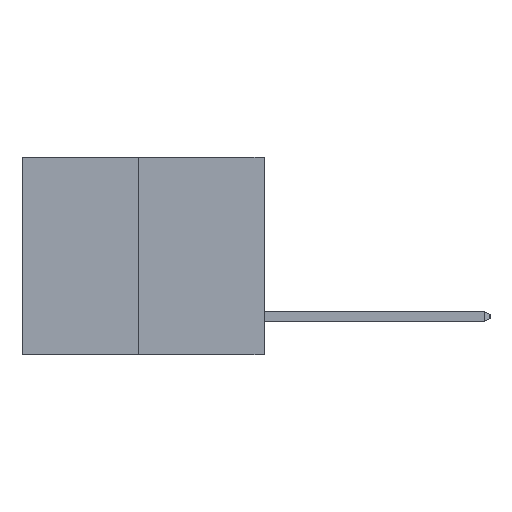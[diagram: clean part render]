
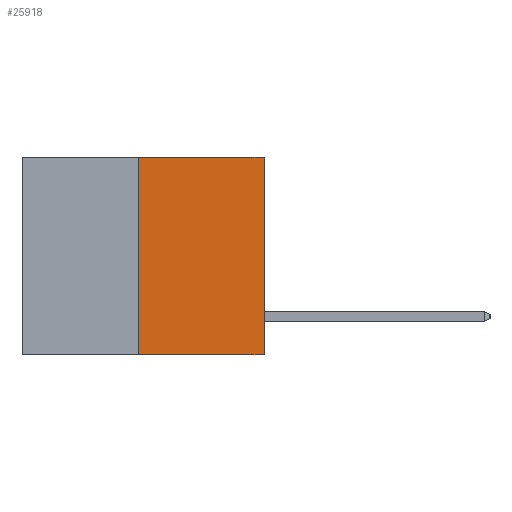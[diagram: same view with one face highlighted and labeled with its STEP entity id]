
A CAD part, left-side view. The second image highlights one B-rep face of the part: STEP entity #25918.
In plain terms, the highlighted planar face has unit normal (-1, 0, 0).
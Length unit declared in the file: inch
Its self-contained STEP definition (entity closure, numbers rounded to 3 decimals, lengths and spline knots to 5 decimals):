
#347 = EDGE_CURVE ( 'NONE', #13254, #6863, #13673, .T. ) ;
#602 = EDGE_CURVE ( 'NONE', #24014, #6863, #19933, .T. ) ;
#3630 = FACE_OUTER_BOUND ( 'NONE', #6779, .T. ) ;
#3712 = CARTESIAN_POINT ( 'NONE',  ( 0., 0.6, -0.49 ) ) ;
#3800 = VECTOR ( 'NONE', #10921, 39.37008 ) ;
#4757 = CARTESIAN_POINT ( 'NONE',  ( 0., 0., 0. ) ) ;
#5006 = CARTESIAN_POINT ( 'NONE',  ( 0., 0.312, 0. ) ) ;
#5652 = PLANE ( 'NONE',  #18351 ) ;
#6779 = EDGE_LOOP ( 'NONE', ( #8605, #16521, #17600, #12822 ) ) ;
#6863 = VERTEX_POINT ( 'NONE', #4757 ) ;
#7067 = CARTESIAN_POINT ( 'NONE',  ( 0., 0.312, -0.49 ) ) ;
#7430 = VECTOR ( 'NONE', #17820, 39.37008 ) ;
#7860 = DIRECTION ( 'NONE',  ( 0., -1., 0. ) ) ;
#8605 = ORIENTED_EDGE ( 'NONE', *, *, #10778, .F. ) ;
#9129 = DIRECTION ( 'NONE',  ( 0., -1., 0. ) ) ;
#10778 = EDGE_CURVE ( 'NONE', #15456, #24014, #16385, .T. ) ;
#10921 = DIRECTION ( 'NONE',  ( 0., 0., 1. ) ) ;
#11393 = CARTESIAN_POINT ( 'NONE',  ( 0., 0.6, 0. ) ) ;
#11877 = CARTESIAN_POINT ( 'NONE',  ( 0., 0., -0.49 ) ) ;
#11909 = DIRECTION ( 'NONE',  ( 0., 0., -1. ) ) ;
#12227 = EDGE_CURVE ( 'NONE', #15456, #13254, #23102, .T. ) ;
#12822 = ORIENTED_EDGE ( 'NONE', *, *, #602, .F. ) ;
#12825 = VECTOR ( 'NONE', #7860, 39.37008 ) ;
#13254 = VERTEX_POINT ( 'NONE', #11877 ) ;
#13673 = LINE ( 'NONE', #23716, #7430 ) ;
#15456 = VERTEX_POINT ( 'NONE', #25842 ) ;
#16385 = LINE ( 'NONE', #7067, #3800 ) ;
#16521 = ORIENTED_EDGE ( 'NONE', *, *, #12227, .T. ) ;
#17600 = ORIENTED_EDGE ( 'NONE', *, *, #347, .T. ) ;
#17614 = CARTESIAN_POINT ( 'NONE',  ( 0., 0.6, 0. ) ) ;
#17820 = DIRECTION ( 'NONE',  ( 0., 0., 1. ) ) ;
#18351 = AXIS2_PLACEMENT_3D ( 'NONE', #17614, #25591, #11909 ) ;
#19933 = LINE ( 'NONE', #11393, #23659 ) ;
#23102 = LINE ( 'NONE', #3712, #12825 ) ;
#23659 = VECTOR ( 'NONE', #9129, 39.37008 ) ;
#23716 = CARTESIAN_POINT ( 'NONE',  ( 0., 0., 0. ) ) ;
#24014 = VERTEX_POINT ( 'NONE', #5006 ) ;
#25591 = DIRECTION ( 'NONE',  ( 1., 0., 0. ) ) ;
#25842 = CARTESIAN_POINT ( 'NONE',  ( 0., 0.312, -0.49 ) ) ;
#25918 = ADVANCED_FACE ( 'NONE', ( #3630 ), #5652, .F. ) ;
